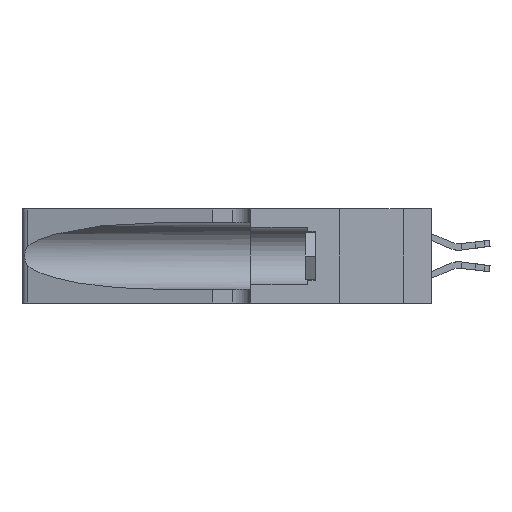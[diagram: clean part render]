
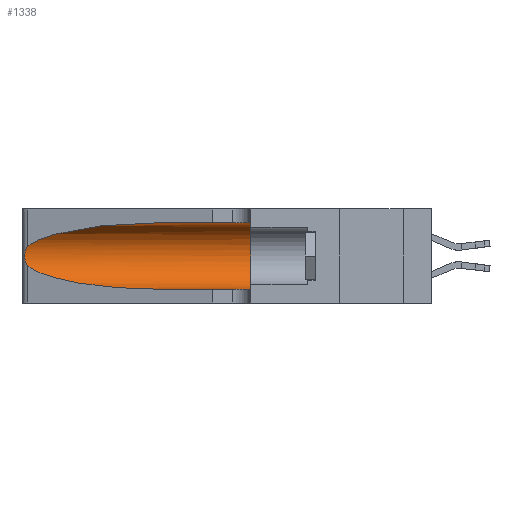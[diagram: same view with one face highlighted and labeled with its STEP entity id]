
A CAD part, left-side view. The second image highlights one B-rep face of the part: STEP entity #1338.
In plain terms, the highlighted cylindrical face has radius 3.308 mm (diameter 6.617 mm), a partial arc.
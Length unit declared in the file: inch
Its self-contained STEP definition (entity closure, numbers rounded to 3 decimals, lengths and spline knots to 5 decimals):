
#273 = VERTEX_POINT ( 'NONE', #19085 ) ;
#731 = B_SPLINE_CURVE_WITH_KNOTS ( 'NONE', 3,
 ( #15970, #17929, #5908, #19878, #8000, #21792, #10064, #23747, #12054, #25703, #14089, #1866, #16048, #3956 ),
 .UNSPECIFIED., .F., .F.,
 ( 4, 2, 2, 2, 2, 2, 4 ),
 ( 0., 0.00027, 0.00053, 0.00107, 0.0016, 0.00187, 0.00214 ),
 .UNSPECIFIED. ) ;
#1290 = AXIS2_PLACEMENT_3D ( 'NONE', #18163, #6180, #20117 ) ;
#1338 = ADVANCED_FACE ( 'NONE', ( #5581 ), #4958, .F. ) ;
#1390 = VERTEX_POINT ( 'NONE', #13470 ) ;
#1434 = CARTESIAN_POINT ( 'NONE',  ( 0.18966, 0.96281, 0.31525 ) ) ;
#1866 = CARTESIAN_POINT ( 'NONE',  ( 0.25639, 1.23186, 0.15144 ) ) ;
#2606 = ORIENTED_EDGE ( 'NONE', *, *, #8417, .T. ) ;
#2894 = VECTOR ( 'NONE', #24339, 39.37008 ) ;
#3956 = CARTESIAN_POINT ( 'NONE',  ( 0.25487, 1.22718, 0.14631 ) ) ;
#4958 = CYLINDRICAL_SURFACE ( 'NONE', #6043, 0.13025 ) ;
#5107 = DIRECTION ( 'NONE',  ( 0., 0., -1. ) ) ;
#5153 = EDGE_CURVE ( 'NONE', #13386, #8803, #18687, .T. ) ;
#5574 = CARTESIAN_POINT ( 'NONE',  ( 0.2373, 1.15595, 0.28018 ) ) ;
#5581 = FACE_OUTER_BOUND ( 'NONE', #15172, .T. ) ;
#5623 = CIRCLE ( 'NONE', #1290, 0.13025 ) ;
#5908 = CARTESIAN_POINT ( 'NONE',  ( 0.25639, 1.23184, 0.21858 ) ) ;
#6043 = AXIS2_PLACEMENT_3D ( 'NONE', #13216, #17157, #5107 ) ;
#6180 = DIRECTION ( 'NONE',  ( 0., 1., 0. ) ) ;
#7631 = ORIENTED_EDGE ( 'NONE', *, *, #22470, .T. ) ;
#7649 = CARTESIAN_POINT ( 'NONE',  ( 0.25487, 1.22718, 0.22369 ) ) ;
#8000 = CARTESIAN_POINT ( 'NONE',  ( 0.25854, 1.2359, 0.20912 ) ) ;
#8307 = EDGE_CURVE ( 'NONE', #13118, #273, #18305, .T. ) ;
#8417 = EDGE_CURVE ( 'NONE', #13118, #24441, #9497, .T. ) ;
#8803 = VERTEX_POINT ( 'NONE', #10912 ) ;
#9497 =( BOUNDED_CURVE ( )  B_SPLINE_CURVE ( 3, ( #23365, #1434, #5574, #7649 ),
 .UNSPECIFIED., .F., .F. ) 
 B_SPLINE_CURVE_WITH_KNOTS ( ( 4, 4 ),
 ( 1.5708, 2.84003 ),
 .UNSPECIFIED. ) 
 CURVE ( )  GEOMETRIC_REPRESENTATION_ITEM ( )  RATIONAL_B_SPLINE_CURVE ( ( 1., 0.87, 0.87, 1. ) ) 
 REPRESENTATION_ITEM ( '' )  );
#10064 = CARTESIAN_POINT ( 'NONE',  ( 0.26075, 1.23896, 0.19203 ) ) ;
#10302 = CARTESIAN_POINT ( 'NONE',  ( 0.18966, 0.96281, 0.05475 ) ) ;
#10643 = CARTESIAN_POINT ( 'NONE',  ( 0.1305, 1.61858, 0.05475 ) ) ;
#10912 = CARTESIAN_POINT ( 'NONE',  ( 0.1305, 0.72297, 0.05475 ) ) ;
#11295 = CARTESIAN_POINT ( 'NONE',  ( 0.1305, 1.61858, 0.31525 ) ) ;
#12054 = CARTESIAN_POINT ( 'NONE',  ( 0.26017, 1.23833, 0.17102 ) ) ;
#12163 = EDGE_CURVE ( 'NONE', #8803, #1390, #18311, .T. ) ;
#12306 = CARTESIAN_POINT ( 'NONE',  ( 0.1305, 0.72297, 0.05475 ) ) ;
#12957 = ORIENTED_EDGE ( 'NONE', *, *, #12163, .T. ) ;
#13110 = VECTOR ( 'NONE', #17274, 39.37008 ) ;
#13118 = VERTEX_POINT ( 'NONE', #13711 ) ;
#13216 = CARTESIAN_POINT ( 'NONE',  ( 0.1305, 1.61858, 0.185 ) ) ;
#13386 = VERTEX_POINT ( 'NONE', #18391 ) ;
#13470 = CARTESIAN_POINT ( 'NONE',  ( 0.1305, 0.35, 0.05475 ) ) ;
#13711 = CARTESIAN_POINT ( 'NONE',  ( 0.1305, 0.72297, 0.31525 ) ) ;
#14089 = CARTESIAN_POINT ( 'NONE',  ( 0.25789, 1.23486, 0.15765 ) ) ;
#15172 = EDGE_LOOP ( 'NONE', ( #2606, #7631, #16831, #12957, #21100, #17656 ) ) ;
#15970 = CARTESIAN_POINT ( 'NONE',  ( 0.25487, 1.22718, 0.22369 ) ) ;
#16048 = CARTESIAN_POINT ( 'NONE',  ( 0.25555, 1.22993, 0.14849 ) ) ;
#16831 = ORIENTED_EDGE ( 'NONE', *, *, #5153, .T. ) ;
#17157 = DIRECTION ( 'NONE',  ( 0., -1., 0. ) ) ;
#17274 = DIRECTION ( 'NONE',  ( 0., -1., 0. ) ) ;
#17656 = ORIENTED_EDGE ( 'NONE', *, *, #8307, .F. ) ;
#17929 = CARTESIAN_POINT ( 'NONE',  ( 0.25555, 1.22994, 0.2215 ) ) ;
#18163 = CARTESIAN_POINT ( 'NONE',  ( 0.1305, 0.35, 0.185 ) ) ;
#18305 = LINE ( 'NONE', #11295, #13110 ) ;
#18311 = LINE ( 'NONE', #10643, #2894 ) ;
#18391 = CARTESIAN_POINT ( 'NONE',  ( 0.25487, 1.22718, 0.14631 ) ) ;
#18687 =( BOUNDED_CURVE ( )  B_SPLINE_CURVE ( 3, ( #23988, #22032, #10302, #12306 ),
 .UNSPECIFIED., .F., .F. ) 
 B_SPLINE_CURVE_WITH_KNOTS ( ( 4, 4 ),
 ( 3.44316, 4.71239 ),
 .UNSPECIFIED. ) 
 CURVE ( )  GEOMETRIC_REPRESENTATION_ITEM ( )  RATIONAL_B_SPLINE_CURVE ( ( 1., 0.87, 0.87, 1. ) ) 
 REPRESENTATION_ITEM ( '' )  );
#19085 = CARTESIAN_POINT ( 'NONE',  ( 0.1305, 0.35, 0.31525 ) ) ;
#19873 = EDGE_CURVE ( 'NONE', #273, #1390, #5623, .T. ) ;
#19878 = CARTESIAN_POINT ( 'NONE',  ( 0.25787, 1.23484, 0.2124 ) ) ;
#20117 = DIRECTION ( 'NONE',  ( 0., 0., 1. ) ) ;
#21100 = ORIENTED_EDGE ( 'NONE', *, *, #19873, .F. ) ;
#21792 = CARTESIAN_POINT ( 'NONE',  ( 0.26018, 1.23835, 0.19895 ) ) ;
#22032 = CARTESIAN_POINT ( 'NONE',  ( 0.2373, 1.15595, 0.08982 ) ) ;
#22470 = EDGE_CURVE ( 'NONE', #24441, #13386, #731, .T. ) ;
#23365 = CARTESIAN_POINT ( 'NONE',  ( 0.1305, 0.72297, 0.31525 ) ) ;
#23747 = CARTESIAN_POINT ( 'NONE',  ( 0.26075, 1.23896, 0.178 ) ) ;
#23988 = CARTESIAN_POINT ( 'NONE',  ( 0.25487, 1.22718, 0.14631 ) ) ;
#24095 = CARTESIAN_POINT ( 'NONE',  ( 0.25487, 1.22718, 0.22369 ) ) ;
#24339 = DIRECTION ( 'NONE',  ( 0., -1., 0. ) ) ;
#24441 = VERTEX_POINT ( 'NONE', #24095 ) ;
#25703 = CARTESIAN_POINT ( 'NONE',  ( 0.25856, 1.23593, 0.16098 ) ) ;
